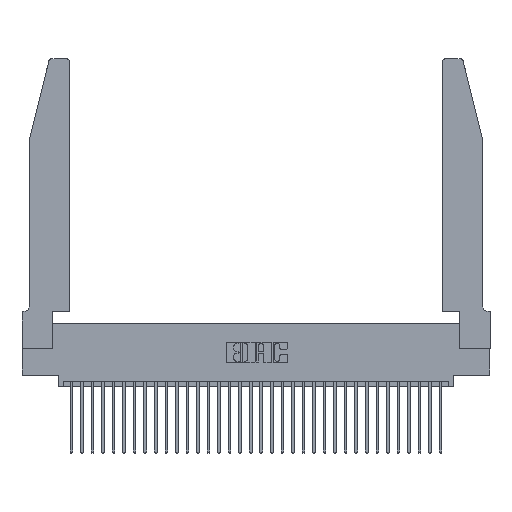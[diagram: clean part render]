
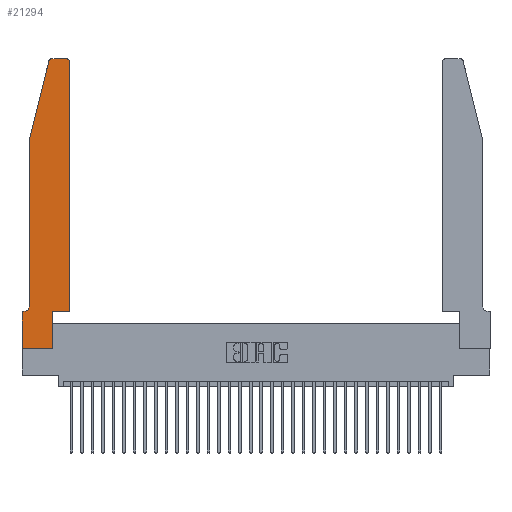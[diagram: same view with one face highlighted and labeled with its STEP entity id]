
A CAD part, top view. The second image highlights one B-rep face of the part: STEP entity #21294.
In plain terms, the highlighted planar face has unit normal (0, 0, 1).
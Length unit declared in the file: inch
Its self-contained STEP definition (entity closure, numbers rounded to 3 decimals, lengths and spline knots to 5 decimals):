
#48 = DIRECTION ( 'NONE',  ( 1., 0., 0. ) ) ;
#123 = CARTESIAN_POINT ( 'NONE',  ( 0.0055, 0.42, 0.37 ) ) ;
#127 = VECTOR ( 'NONE', #11975, 39.37008 ) ;
#162 = CARTESIAN_POINT ( 'NONE',  ( 0.0755, 0.42, 0.37 ) ) ;
#1024 = VERTEX_POINT ( 'NONE', #13404 ) ;
#1189 = VERTEX_POINT ( 'NONE', #24377 ) ;
#1613 = AXIS2_PLACEMENT_3D ( 'NONE', #10235, #28531, #12854 ) ;
#2022 = ORIENTED_EDGE ( 'NONE', *, *, #6634, .T. ) ;
#2780 = DIRECTION ( 'NONE',  ( -1., 0., 0. ) ) ;
#3210 = CARTESIAN_POINT ( 'NONE',  ( 0.284, 2.75, 0.37 ) ) ;
#3302 = CIRCLE ( 'NONE', #12170, 0.03 ) ;
#3318 = ORIENTED_EDGE ( 'NONE', *, *, #27943, .T. ) ;
#3792 = EDGE_CURVE ( 'NONE', #18438, #16917, #9145, .T. ) ;
#3963 = VECTOR ( 'NONE', #16347, 39.37008 ) ;
#4232 = VECTOR ( 'NONE', #4814, 39.37008 ) ;
#4379 = CARTESIAN_POINT ( 'NONE',  ( 0., 0.35, 0.37 ) ) ;
#4814 = DIRECTION ( 'NONE',  ( -1., 0., 0. ) ) ;
#4934 = CARTESIAN_POINT ( 'NONE',  ( 0.4505, 0.35, 0.37 ) ) ;
#5854 = CARTESIAN_POINT ( 'NONE',  ( 0.4205, 2.75, 0.37 ) ) ;
#6634 = EDGE_CURVE ( 'NONE', #30984, #10936, #22883, .T. ) ;
#6716 = CARTESIAN_POINT ( 'NONE',  ( 0.25487, 2.72718, 0.37 ) ) ;
#6744 = VECTOR ( 'NONE', #17628, 39.37008 ) ;
#7142 = LINE ( 'NONE', #9344, #127 ) ;
#7479 = FACE_OUTER_BOUND ( 'NONE', #7569, .T. ) ;
#7569 = EDGE_LOOP ( 'NONE', ( #32809, #12761, #28320, #2022, #29974, #10736, #33226, #21032, #22642, #3318, #32032, #11977 ) ) ;
#7866 = AXIS2_PLACEMENT_3D ( 'NONE', #24736, #24847, #9158 ) ;
#8006 = VECTOR ( 'NONE', #29571, 39.37008 ) ;
#8292 = EDGE_CURVE ( 'NONE', #28817, #25919, #28472, .T. ) ;
#8370 = EDGE_CURVE ( 'NONE', #16917, #12250, #25208, .T. ) ;
#8856 = VECTOR ( 'NONE', #11875, 39.37008 ) ;
#9145 = CIRCLE ( 'NONE', #1613, 0.03 ) ;
#9158 = DIRECTION ( 'NONE',  ( 1., 0., 0. ) ) ;
#9237 = CARTESIAN_POINT ( 'NONE',  ( 0.0755, 2., 0.37 ) ) ;
#9344 = CARTESIAN_POINT ( 'NONE',  ( 0., 0., 0.37 ) ) ;
#9894 = CARTESIAN_POINT ( 'NONE',  ( 0.0755, 2., 0.37 ) ) ;
#10075 = EDGE_CURVE ( 'NONE', #15629, #30984, #30526, .T. ) ;
#10235 = CARTESIAN_POINT ( 'NONE',  ( 0.4205, 2.72, 0.37 ) ) ;
#10736 = ORIENTED_EDGE ( 'NONE', *, *, #8292, .T. ) ;
#10936 = VERTEX_POINT ( 'NONE', #162 ) ;
#11059 = CARTESIAN_POINT ( 'NONE',  ( 0., 0., 0.37 ) ) ;
#11539 = CARTESIAN_POINT ( 'NONE',  ( 0.4505, 0.35, 0.37 ) ) ;
#11549 = EDGE_CURVE ( 'NONE', #10936, #28817, #15747, .T. ) ;
#11875 = DIRECTION ( 'NONE',  ( -0.239, -0.971, 0. ) ) ;
#11975 = DIRECTION ( 'NONE',  ( 1., 0., 0. ) ) ;
#11977 = ORIENTED_EDGE ( 'NONE', *, *, #3792, .T. ) ;
#12170 = AXIS2_PLACEMENT_3D ( 'NONE', #31484, #15853, #48 ) ;
#12250 = VERTEX_POINT ( 'NONE', #3210 ) ;
#12259 = VECTOR ( 'NONE', #18000, 39.37008 ) ;
#12761 = ORIENTED_EDGE ( 'NONE', *, *, #33824, .T. ) ;
#12854 = DIRECTION ( 'NONE',  ( 1., 0., 0. ) ) ;
#13404 = CARTESIAN_POINT ( 'NONE',  ( 0.2865, 0.35, 0.37 ) ) ;
#13777 = EDGE_CURVE ( 'NONE', #19997, #18438, #19292, .T. ) ;
#14212 = CARTESIAN_POINT ( 'NONE',  ( 0.0055, 0.35, 0.37 ) ) ;
#15629 = VERTEX_POINT ( 'NONE', #6716 ) ;
#15747 = CIRCLE ( 'NONE', #21581, 0.07 ) ;
#15853 = DIRECTION ( 'NONE',  ( 0., 0., 1. ) ) ;
#16347 = DIRECTION ( 'NONE',  ( 0., -1., 0. ) ) ;
#16917 = VERTEX_POINT ( 'NONE', #5854 ) ;
#17628 = DIRECTION ( 'NONE',  ( -1., 0., 0. ) ) ;
#18000 = DIRECTION ( 'NONE',  ( 0., 1., 0. ) ) ;
#18438 = VERTEX_POINT ( 'NONE', #20258 ) ;
#18580 = DIRECTION ( 'NONE',  ( 0., 0., -1. ) ) ;
#19292 = LINE ( 'NONE', #25751, #12259 ) ;
#19997 = VERTEX_POINT ( 'NONE', #11539 ) ;
#20124 = EDGE_CURVE ( 'NONE', #26320, #1189, #7142, .T. ) ;
#20258 = CARTESIAN_POINT ( 'NONE',  ( 0.4505, 2.72, 0.37 ) ) ;
#21032 = ORIENTED_EDGE ( 'NONE', *, *, #20124, .T. ) ;
#21294 = ADVANCED_FACE ( 'NONE', ( #7479 ), #22234, .T. ) ;
#21581 = AXIS2_PLACEMENT_3D ( 'NONE', #123, #18580, #2780 ) ;
#22088 = VECTOR ( 'NONE', #30804, 39.37008 ) ;
#22234 = PLANE ( 'NONE',  #7866 ) ;
#22332 = CARTESIAN_POINT ( 'NONE',  ( 0., 0., 0.37 ) ) ;
#22642 = ORIENTED_EDGE ( 'NONE', *, *, #31618, .T. ) ;
#22883 = LINE ( 'NONE', #9894, #22088 ) ;
#23328 = DIRECTION ( 'NONE',  ( 1., 0., 0. ) ) ;
#24377 = CARTESIAN_POINT ( 'NONE',  ( 0.2865, 0., 0.37 ) ) ;
#24736 = CARTESIAN_POINT ( 'NONE',  ( 0., 0.35, 0.37 ) ) ;
#24789 = VECTOR ( 'NONE', #23328, 39.37008 ) ;
#24847 = DIRECTION ( 'NONE',  ( 0., 0., 1. ) ) ;
#24989 = EDGE_CURVE ( 'NONE', #25919, #26320, #31872, .T. ) ;
#25208 = LINE ( 'NONE', #33598, #4232 ) ;
#25599 = LINE ( 'NONE', #4934, #24789 ) ;
#25751 = CARTESIAN_POINT ( 'NONE',  ( 0.4505, 0.35, 0.37 ) ) ;
#25919 = VERTEX_POINT ( 'NONE', #4379 ) ;
#26320 = VERTEX_POINT ( 'NONE', #22332 ) ;
#26955 = CARTESIAN_POINT ( 'NONE',  ( 0.2865, 0.35, 0.37 ) ) ;
#27943 = EDGE_CURVE ( 'NONE', #1024, #19997, #25599, .T. ) ;
#27993 = CARTESIAN_POINT ( 'NONE',  ( 0.0755, 0.35, 0.37 ) ) ;
#28320 = ORIENTED_EDGE ( 'NONE', *, *, #10075, .T. ) ;
#28472 = LINE ( 'NONE', #27993, #6744 ) ;
#28531 = DIRECTION ( 'NONE',  ( 0., 0., 1. ) ) ;
#28817 = VERTEX_POINT ( 'NONE', #14212 ) ;
#28912 = LINE ( 'NONE', #26955, #8006 ) ;
#29571 = DIRECTION ( 'NONE',  ( 0., 1., 0. ) ) ;
#29974 = ORIENTED_EDGE ( 'NONE', *, *, #11549, .T. ) ;
#30526 = LINE ( 'NONE', #9237, #8856 ) ;
#30804 = DIRECTION ( 'NONE',  ( 0., -1., 0. ) ) ;
#30984 = VERTEX_POINT ( 'NONE', #32338 ) ;
#31484 = CARTESIAN_POINT ( 'NONE',  ( 0.284, 2.72, 0.37 ) ) ;
#31618 = EDGE_CURVE ( 'NONE', #1189, #1024, #28912, .T. ) ;
#31872 = LINE ( 'NONE', #11059, #3963 ) ;
#32032 = ORIENTED_EDGE ( 'NONE', *, *, #13777, .T. ) ;
#32338 = CARTESIAN_POINT ( 'NONE',  ( 0.0755, 2., 0.37 ) ) ;
#32809 = ORIENTED_EDGE ( 'NONE', *, *, #8370, .T. ) ;
#33226 = ORIENTED_EDGE ( 'NONE', *, *, #24989, .T. ) ;
#33598 = CARTESIAN_POINT ( 'NONE',  ( 0.2605, 2.75, 0.37 ) ) ;
#33824 = EDGE_CURVE ( 'NONE', #12250, #15629, #3302, .T. ) ;
